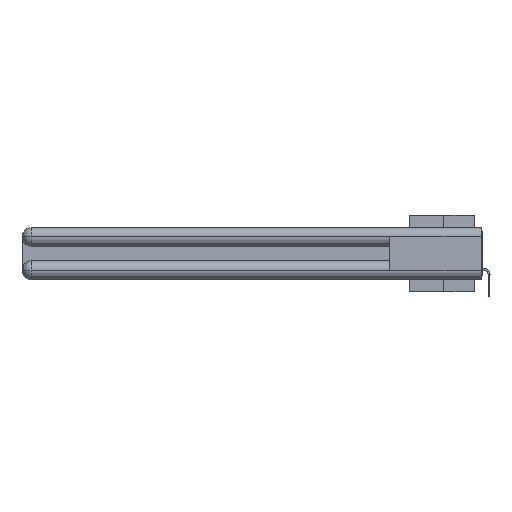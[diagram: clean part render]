
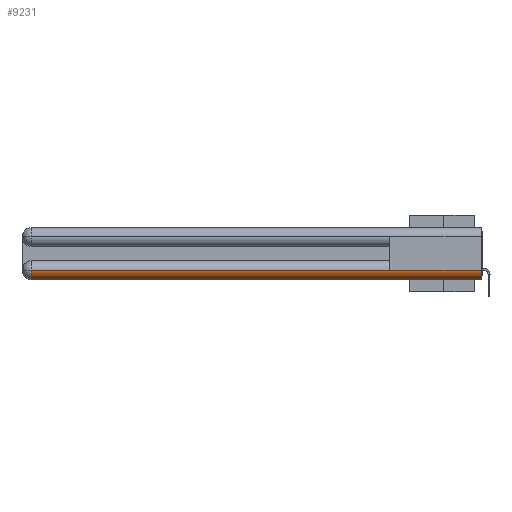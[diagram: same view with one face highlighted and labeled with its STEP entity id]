
A CAD part, left-side view. The second image highlights one B-rep face of the part: STEP entity #9231.
In plain terms, the highlighted cylindrical face has radius 1.562 mm (diameter 3.124 mm), a partial arc.
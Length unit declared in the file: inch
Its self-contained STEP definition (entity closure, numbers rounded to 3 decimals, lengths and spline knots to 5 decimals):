
#388 = CARTESIAN_POINT ( 'NONE',  ( 0., 0.6, -0.2785 ) ) ;
#582 = LINE ( 'NONE', #8003, #7073 ) ;
#3344 = CIRCLE ( 'NONE', #9916, 0.0615 ) ;
#3479 = AXIS2_PLACEMENT_3D ( 'NONE', #14302, #21783, #12537 ) ;
#4666 = EDGE_CURVE ( 'NONE', #27969, #10148, #582, .T. ) ;
#5207 = ORIENTED_EDGE ( 'NONE', *, *, #26871, .F. ) ;
#5594 = VERTEX_POINT ( 'NONE', #18147 ) ;
#7073 = VECTOR ( 'NONE', #19973, 39.37008 ) ;
#7082 = FACE_OUTER_BOUND ( 'NONE', #23832, .T. ) ;
#7837 = DIRECTION ( 'NONE',  ( 0., -1., 0. ) ) ;
#8003 = CARTESIAN_POINT ( 'NONE',  ( 0., 0., -0.2785 ) ) ;
#8577 = VECTOR ( 'NONE', #29935, 39.37008 ) ;
#8841 = DIRECTION ( 'NONE',  ( 0., 1., 0. ) ) ;
#9231 = ADVANCED_FACE ( 'NONE', ( #7082 ), #31438, .T. ) ;
#9467 = CARTESIAN_POINT ( 'NONE',  ( 0.0615, 0., -0.34 ) ) ;
#9916 = AXIS2_PLACEMENT_3D ( 'NONE', #29658, #7837, #30290 ) ;
#10148 = VERTEX_POINT ( 'NONE', #25818 ) ;
#10341 = CARTESIAN_POINT ( 'NONE',  ( 0., 0., -0.2785 ) ) ;
#10820 = AXIS2_PLACEMENT_3D ( 'NONE', #23236, #21434, #26844 ) ;
#12084 = CIRCLE ( 'NONE', #3479, 0.0615 ) ;
#12367 = EDGE_CURVE ( 'NONE', #5594, #22569, #31135, .T. ) ;
#12537 = DIRECTION ( 'NONE',  ( 1., 0., 0. ) ) ;
#13123 = EDGE_CURVE ( 'NONE', #22334, #22569, #3344, .T. ) ;
#14302 = CARTESIAN_POINT ( 'NONE',  ( 0.0615, 0., -0.2785 ) ) ;
#15625 = CARTESIAN_POINT ( 'NONE',  ( 0., 2.94, -0.2785 ) ) ;
#15840 = ORIENTED_EDGE ( 'NONE', *, *, #18156, .T. ) ;
#17999 = ORIENTED_EDGE ( 'NONE', *, *, #4666, .F. ) ;
#18147 = CARTESIAN_POINT ( 'NONE',  ( 0.0615, 0., -0.34 ) ) ;
#18156 = EDGE_CURVE ( 'NONE', #27969, #22334, #22311, .T. ) ;
#19382 = ORIENTED_EDGE ( 'NONE', *, *, #13123, .T. ) ;
#19694 = CARTESIAN_POINT ( 'NONE',  ( 0.0615, 2.94, -0.34 ) ) ;
#19973 = DIRECTION ( 'NONE',  ( 0., -1., 0. ) ) ;
#21434 = DIRECTION ( 'NONE',  ( 0., -1., 0. ) ) ;
#21783 = DIRECTION ( 'NONE',  ( 0., -1., 0. ) ) ;
#22311 = LINE ( 'NONE', #10341, #8577 ) ;
#22334 = VERTEX_POINT ( 'NONE', #15625 ) ;
#22569 = VERTEX_POINT ( 'NONE', #19694 ) ;
#23236 = CARTESIAN_POINT ( 'NONE',  ( 0.0615, 0., -0.2785 ) ) ;
#23832 = EDGE_LOOP ( 'NONE', ( #15840, #19382, #26469, #5207, #17999 ) ) ;
#25818 = CARTESIAN_POINT ( 'NONE',  ( 0., 0., -0.2785 ) ) ;
#26469 = ORIENTED_EDGE ( 'NONE', *, *, #12367, .F. ) ;
#26844 = DIRECTION ( 'NONE',  ( 0., 0., -1. ) ) ;
#26871 = EDGE_CURVE ( 'NONE', #10148, #5594, #12084, .T. ) ;
#27969 = VERTEX_POINT ( 'NONE', #388 ) ;
#29658 = CARTESIAN_POINT ( 'NONE',  ( 0.0615, 2.94, -0.2785 ) ) ;
#29935 = DIRECTION ( 'NONE',  ( 0., 1., 0. ) ) ;
#30290 = DIRECTION ( 'NONE',  ( 0., 0., 1. ) ) ;
#31135 = LINE ( 'NONE', #9467, #31234 ) ;
#31234 = VECTOR ( 'NONE', #8841, 39.37008 ) ;
#31438 = CYLINDRICAL_SURFACE ( 'NONE', #10820, 0.0615 ) ;
